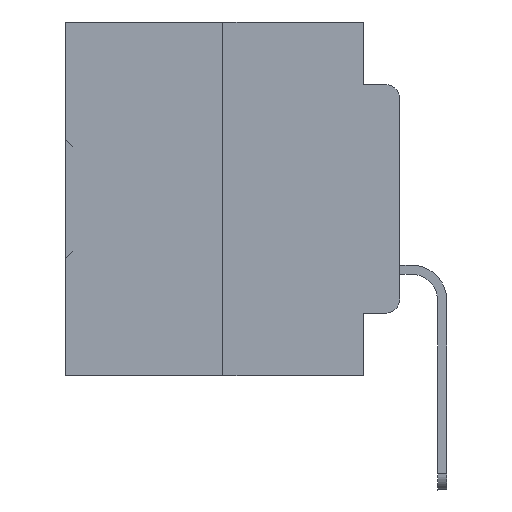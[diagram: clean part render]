
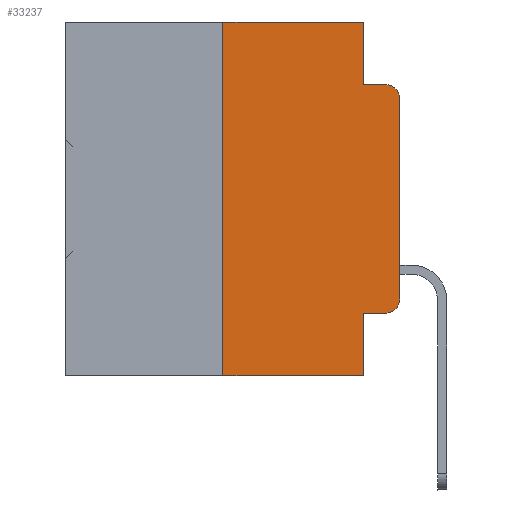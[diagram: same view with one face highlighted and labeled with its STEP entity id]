
A CAD part, left-side view. The second image highlights one B-rep face of the part: STEP entity #33237.
In plain terms, the highlighted planar face has unit normal (-1, 0, 0).
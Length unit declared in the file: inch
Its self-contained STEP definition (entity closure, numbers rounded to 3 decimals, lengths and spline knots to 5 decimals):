
#893 = DIRECTION ( 'NONE',  ( 0., 0., -1. ) ) ;
#956 = EDGE_CURVE ( 'NONE', #26121, #34841, #12850, .T. ) ;
#1041 = ORIENTED_EDGE ( 'NONE', *, *, #34557, .T. ) ;
#1085 = ORIENTED_EDGE ( 'NONE', *, *, #956, .F. ) ;
#1303 = DIRECTION ( 'NONE',  ( 0., 0., -1. ) ) ;
#1665 = CARTESIAN_POINT ( 'NONE',  ( 0., 0.02, -0.0885 ) ) ;
#1901 = VERTEX_POINT ( 'NONE', #7618 ) ;
#1914 = DIRECTION ( 'NONE',  ( 0., -1., 0. ) ) ;
#2435 = VERTEX_POINT ( 'NONE', #1665 ) ;
#3405 = EDGE_CURVE ( 'NONE', #18614, #7851, #11386, .T. ) ;
#3714 = LINE ( 'NONE', #24649, #5264 ) ;
#4120 = EDGE_CURVE ( 'NONE', #37113, #5837, #28294, .T. ) ;
#4417 = CARTESIAN_POINT ( 'NONE',  ( 0., 0.051, -0.4115 ) ) ;
#5170 = ORIENTED_EDGE ( 'NONE', *, *, #4120, .T. ) ;
#5264 = VECTOR ( 'NONE', #36626, 39.37008 ) ;
#5354 = VECTOR ( 'NONE', #34894, 39.37008 ) ;
#5837 = VERTEX_POINT ( 'NONE', #31196 ) ;
#5981 = CARTESIAN_POINT ( 'NONE',  ( 0., 0.051, -0.0885 ) ) ;
#7352 = VECTOR ( 'NONE', #31811, 39.37008 ) ;
#7618 = CARTESIAN_POINT ( 'NONE',  ( 0., 0.051, 0. ) ) ;
#7851 = VERTEX_POINT ( 'NONE', #7949 ) ;
#7949 = CARTESIAN_POINT ( 'NONE',  ( 0., 0., -0.1085 ) ) ;
#9093 = ORIENTED_EDGE ( 'NONE', *, *, #25690, .T. ) ;
#10317 = CARTESIAN_POINT ( 'NONE',  ( 0., 0.02, -0.1085 ) ) ;
#10669 = CARTESIAN_POINT ( 'NONE',  ( 0., 0.051, -0.4115 ) ) ;
#11194 = CARTESIAN_POINT ( 'NONE',  ( 0., 0., 0. ) ) ;
#11368 = DIRECTION ( 'NONE',  ( -1., 0., 0. ) ) ;
#11386 = LINE ( 'NONE', #11194, #5354 ) ;
#12292 = VECTOR ( 'NONE', #18468, 39.37008 ) ;
#12783 = CIRCLE ( 'NONE', #29679, 0.02 ) ;
#12850 = LINE ( 'NONE', #21661, #36450 ) ;
#13245 = CARTESIAN_POINT ( 'NONE',  ( 0., 0.473, 0. ) ) ;
#14557 = LINE ( 'NONE', #35348, #38597 ) ;
#15520 = EDGE_CURVE ( 'NONE', #34841, #1901, #19721, .T. ) ;
#15556 = LINE ( 'NONE', #5981, #23112 ) ;
#17550 = EDGE_CURVE ( 'NONE', #31810, #2435, #15556, .T. ) ;
#18298 = DIRECTION ( 'NONE',  ( 0., -1., 0. ) ) ;
#18468 = DIRECTION ( 'NONE',  ( 0., 0., -1. ) ) ;
#18614 = VERTEX_POINT ( 'NONE', #21932 ) ;
#19721 = LINE ( 'NONE', #37770, #37484 ) ;
#20638 = CARTESIAN_POINT ( 'NONE',  ( 0., 0.25, 0. ) ) ;
#20836 = AXIS2_PLACEMENT_3D ( 'NONE', #13245, #36984, #893 ) ;
#21661 = CARTESIAN_POINT ( 'NONE',  ( 0., 0.25, 0. ) ) ;
#21929 = ORIENTED_EDGE ( 'NONE', *, *, #28797, .F. ) ;
#21932 = CARTESIAN_POINT ( 'NONE',  ( 0., 0., -0.3915 ) ) ;
#23112 = VECTOR ( 'NONE', #18298, 39.37008 ) ;
#23355 = CIRCLE ( 'NONE', #29635, 0.02 ) ;
#23953 = ORIENTED_EDGE ( 'NONE', *, *, #30144, .F. ) ;
#23967 = LINE ( 'NONE', #30646, #12292 ) ;
#23971 = CARTESIAN_POINT ( 'NONE',  ( 0., 0.051, -0.0885 ) ) ;
#24649 = CARTESIAN_POINT ( 'NONE',  ( 0., 0.473, -0.5 ) ) ;
#25261 = CARTESIAN_POINT ( 'NONE',  ( 0., 0.051, -0.5 ) ) ;
#25690 = EDGE_CURVE ( 'NONE', #5837, #18614, #23355, .T. ) ;
#26121 = VERTEX_POINT ( 'NONE', #37585 ) ;
#26161 = ORIENTED_EDGE ( 'NONE', *, *, #34109, .T. ) ;
#26333 = DIRECTION ( 'NONE',  ( 0., 0., -1. ) ) ;
#27531 = EDGE_LOOP ( 'NONE', ( #31228, #1041, #31613, #21929, #32683, #1085, #26161, #23953, #5170, #9093 ) ) ;
#28294 = LINE ( 'NONE', #10669, #7352 ) ;
#28797 = EDGE_CURVE ( 'NONE', #1901, #31810, #14557, .T. ) ;
#29175 = CARTESIAN_POINT ( 'NONE',  ( 0., 0.02, -0.3915 ) ) ;
#29635 = AXIS2_PLACEMENT_3D ( 'NONE', #29175, #11368, #35460 ) ;
#29679 = AXIS2_PLACEMENT_3D ( 'NONE', #10317, #33851, #1303 ) ;
#30144 = EDGE_CURVE ( 'NONE', #37113, #31055, #23967, .T. ) ;
#30646 = CARTESIAN_POINT ( 'NONE',  ( 0., 0.051, 0. ) ) ;
#30698 = FACE_OUTER_BOUND ( 'NONE', #27531, .T. ) ;
#31055 = VERTEX_POINT ( 'NONE', #25261 ) ;
#31196 = CARTESIAN_POINT ( 'NONE',  ( 0., 0.02, -0.4115 ) ) ;
#31228 = ORIENTED_EDGE ( 'NONE', *, *, #3405, .T. ) ;
#31613 = ORIENTED_EDGE ( 'NONE', *, *, #17550, .F. ) ;
#31810 = VERTEX_POINT ( 'NONE', #23971 ) ;
#31811 = DIRECTION ( 'NONE',  ( 0., -1., 0. ) ) ;
#32683 = ORIENTED_EDGE ( 'NONE', *, *, #15520, .F. ) ;
#33237 = ADVANCED_FACE ( 'NONE', ( #30698 ), #33843, .F. ) ;
#33644 = DIRECTION ( 'NONE',  ( 0., 0., 1. ) ) ;
#33843 = PLANE ( 'NONE',  #20836 ) ;
#33851 = DIRECTION ( 'NONE',  ( -1., 0., 0. ) ) ;
#34109 = EDGE_CURVE ( 'NONE', #26121, #31055, #3714, .T. ) ;
#34557 = EDGE_CURVE ( 'NONE', #7851, #2435, #12783, .T. ) ;
#34841 = VERTEX_POINT ( 'NONE', #20638 ) ;
#34894 = DIRECTION ( 'NONE',  ( 0., 0., 1. ) ) ;
#35348 = CARTESIAN_POINT ( 'NONE',  ( 0., 0.051, 0. ) ) ;
#35460 = DIRECTION ( 'NONE',  ( 0., 0., -1. ) ) ;
#36450 = VECTOR ( 'NONE', #33644, 39.37008 ) ;
#36626 = DIRECTION ( 'NONE',  ( 0., -1., 0. ) ) ;
#36984 = DIRECTION ( 'NONE',  ( 1., 0., 0. ) ) ;
#37113 = VERTEX_POINT ( 'NONE', #4417 ) ;
#37484 = VECTOR ( 'NONE', #1914, 39.37008 ) ;
#37585 = CARTESIAN_POINT ( 'NONE',  ( 0., 0.25, -0.5 ) ) ;
#37770 = CARTESIAN_POINT ( 'NONE',  ( 0., 0.473, 0. ) ) ;
#38597 = VECTOR ( 'NONE', #26333, 39.37008 ) ;
